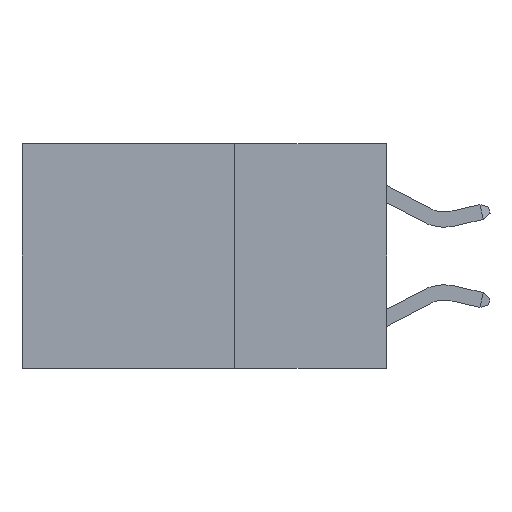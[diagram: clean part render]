
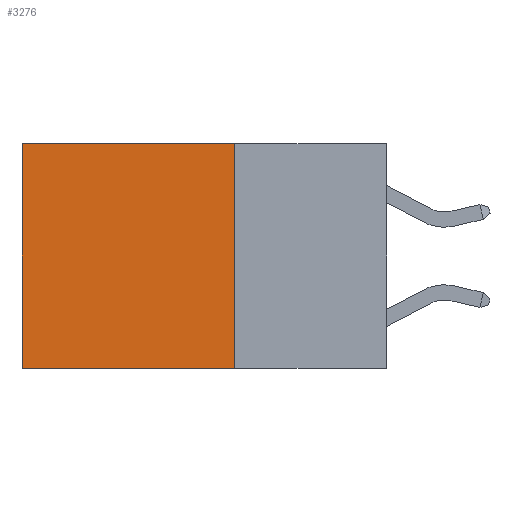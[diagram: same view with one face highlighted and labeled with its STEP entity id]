
A CAD part, left-side view. The second image highlights one B-rep face of the part: STEP entity #3276.
In plain terms, the highlighted planar face has unit normal (-1, 0, 0).
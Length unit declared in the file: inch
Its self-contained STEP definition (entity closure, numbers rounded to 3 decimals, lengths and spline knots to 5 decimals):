
#223 = VERTEX_POINT ( 'NONE', #3098 ) ;
#1330 = LINE ( 'NONE', #3019, #11327 ) ;
#2386 = ORIENTED_EDGE ( 'NONE', *, *, #10054, .F. ) ;
#3019 = CARTESIAN_POINT ( 'NONE',  ( 0.2625, 0.25, -0.37 ) ) ;
#3098 = CARTESIAN_POINT ( 'NONE',  ( 0.2625, 0.25, 0. ) ) ;
#3276 = ADVANCED_FACE ( 'NONE', ( #12052 ), #13899, .F. ) ;
#4297 = DIRECTION ( 'NONE',  ( 0., 1., 0. ) ) ;
#5146 = CARTESIAN_POINT ( 'NONE',  ( 0.2625, 0.6, -0.37 ) ) ;
#5368 = EDGE_CURVE ( 'NONE', #223, #11492, #7637, .T. ) ;
#5772 = DIRECTION ( 'NONE',  ( 0., 0., -1. ) ) ;
#6414 = CARTESIAN_POINT ( 'NONE',  ( 0.2625, 0.6, 0. ) ) ;
#6495 = VECTOR ( 'NONE', #5772, 39.37008 ) ;
#6792 = CARTESIAN_POINT ( 'NONE',  ( 0.2625, 0.25, 0. ) ) ;
#7022 = EDGE_LOOP ( 'NONE', ( #11917, #14893, #2386, #15238 ) ) ;
#7337 = EDGE_CURVE ( 'NONE', #7812, #12294, #1330, .T. ) ;
#7501 = LINE ( 'NONE', #14758, #11469 ) ;
#7637 = LINE ( 'NONE', #9695, #10859 ) ;
#7812 = VERTEX_POINT ( 'NONE', #10410 ) ;
#8067 = DIRECTION ( 'NONE',  ( 0., 0., -1. ) ) ;
#8593 = AXIS2_PLACEMENT_3D ( 'NONE', #6792, #15003, #8067 ) ;
#9425 = LINE ( 'NONE', #14124, #6495 ) ;
#9695 = CARTESIAN_POINT ( 'NONE',  ( 0.2625, 0.25, 0. ) ) ;
#10054 = EDGE_CURVE ( 'NONE', #223, #7812, #7501, .T. ) ;
#10285 = EDGE_CURVE ( 'NONE', #11492, #12294, #9425, .T. ) ;
#10410 = CARTESIAN_POINT ( 'NONE',  ( 0.2625, 0.25, -0.37 ) ) ;
#10859 = VECTOR ( 'NONE', #15374, 39.37008 ) ;
#11327 = VECTOR ( 'NONE', #4297, 39.37008 ) ;
#11353 = DIRECTION ( 'NONE',  ( 0., 0., -1. ) ) ;
#11469 = VECTOR ( 'NONE', #11353, 39.37008 ) ;
#11492 = VERTEX_POINT ( 'NONE', #6414 ) ;
#11917 = ORIENTED_EDGE ( 'NONE', *, *, #10285, .T. ) ;
#12052 = FACE_OUTER_BOUND ( 'NONE', #7022, .T. ) ;
#12294 = VERTEX_POINT ( 'NONE', #5146 ) ;
#13899 = PLANE ( 'NONE',  #8593 ) ;
#14124 = CARTESIAN_POINT ( 'NONE',  ( 0.2625, 0.6, 0. ) ) ;
#14758 = CARTESIAN_POINT ( 'NONE',  ( 0.2625, 0.25, 0. ) ) ;
#14893 = ORIENTED_EDGE ( 'NONE', *, *, #7337, .F. ) ;
#15003 = DIRECTION ( 'NONE',  ( 1., 0., 0. ) ) ;
#15238 = ORIENTED_EDGE ( 'NONE', *, *, #5368, .T. ) ;
#15374 = DIRECTION ( 'NONE',  ( 0., 1., 0. ) ) ;
